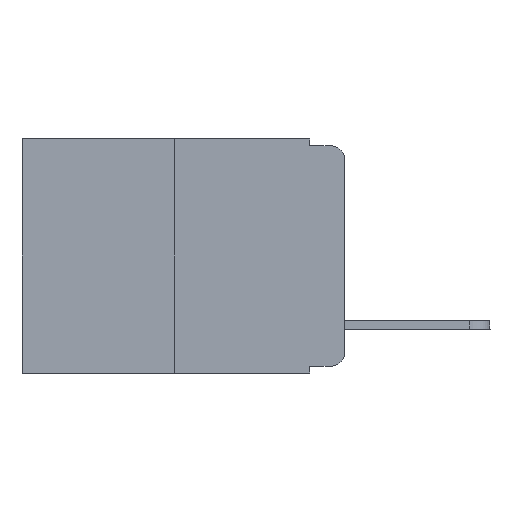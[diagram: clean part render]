
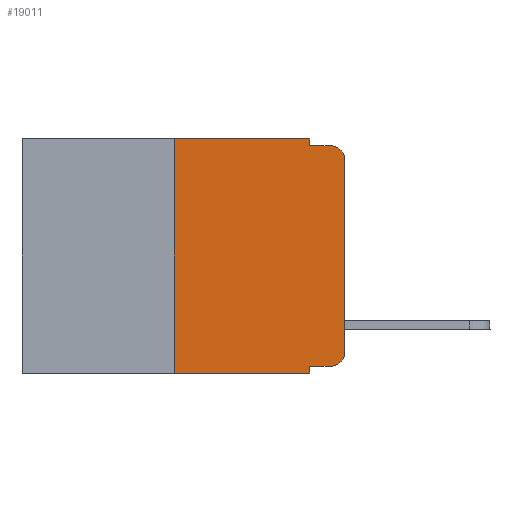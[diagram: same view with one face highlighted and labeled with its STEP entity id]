
A CAD part, left-side view. The second image highlights one B-rep face of the part: STEP entity #19011.
In plain terms, the highlighted planar face has unit normal (-1, 0, 0).
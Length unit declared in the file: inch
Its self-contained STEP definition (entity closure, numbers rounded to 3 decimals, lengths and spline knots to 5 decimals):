
#94 = VERTEX_POINT ( 'NONE', #7996 ) ;
#113 = EDGE_CURVE ( 'NONE', #15430, #3689, #9825, .T. ) ;
#119 = DIRECTION ( 'NONE',  ( -1., 0., 0. ) ) ;
#294 = DIRECTION ( 'NONE',  ( 0., 0., -1. ) ) ;
#566 = CARTESIAN_POINT ( 'NONE',  ( 0., 0.473, 0. ) ) ;
#1064 = ORIENTED_EDGE ( 'NONE', *, *, #1362, .F. ) ;
#1362 = EDGE_CURVE ( 'NONE', #15430, #94, #21019, .T. ) ;
#1914 = CIRCLE ( 'NONE', #5356, 0.02 ) ;
#1919 = CARTESIAN_POINT ( 'NONE',  ( 0., 0.051, 0. ) ) ;
#2071 = VECTOR ( 'NONE', #9882, 39.37008 ) ;
#2117 = VERTEX_POINT ( 'NONE', #2987 ) ;
#2472 = EDGE_CURVE ( 'NONE', #2117, #18087, #5117, .T. ) ;
#2649 = DIRECTION ( 'NONE',  ( 0., 0., 1. ) ) ;
#2950 = EDGE_CURVE ( 'NONE', #3612, #16257, #9960, .T. ) ;
#2987 = CARTESIAN_POINT ( 'NONE',  ( 0., 0.051, -0.01 ) ) ;
#3476 = DIRECTION ( 'NONE',  ( 0., 0., -1. ) ) ;
#3612 = VERTEX_POINT ( 'NONE', #15667 ) ;
#3689 = VERTEX_POINT ( 'NONE', #11002 ) ;
#3691 = VECTOR ( 'NONE', #4846, 39.37008 ) ;
#4055 = VECTOR ( 'NONE', #294, 39.37008 ) ;
#4326 = VECTOR ( 'NONE', #7541, 39.37008 ) ;
#4576 = CARTESIAN_POINT ( 'NONE',  ( 0., 0.473, 0. ) ) ;
#4703 = CARTESIAN_POINT ( 'NONE',  ( 0., 0.25, -0.343 ) ) ;
#4846 = DIRECTION ( 'NONE',  ( 0., -1., 0. ) ) ;
#5110 = EDGE_LOOP ( 'NONE', ( #17208, #15035, #13707, #11684, #19868, #1064, #16160, #17152, #14016, #7458 ) ) ;
#5117 = LINE ( 'NONE', #5328, #2071 ) ;
#5328 = CARTESIAN_POINT ( 'NONE',  ( 0., 0.051, -0.01 ) ) ;
#5356 = AXIS2_PLACEMENT_3D ( 'NONE', #14926, #119, #3476 ) ;
#6059 = CARTESIAN_POINT ( 'NONE',  ( 0., 0., -0.03 ) ) ;
#6173 = CARTESIAN_POINT ( 'NONE',  ( 0., 0.25, 0. ) ) ;
#6308 = EDGE_CURVE ( 'NONE', #16737, #3689, #9703, .T. ) ;
#6925 = LINE ( 'NONE', #566, #19804 ) ;
#7283 = VERTEX_POINT ( 'NONE', #10269 ) ;
#7458 = ORIENTED_EDGE ( 'NONE', *, *, #16545, .T. ) ;
#7541 = DIRECTION ( 'NONE',  ( 0., 0., -1. ) ) ;
#7996 = CARTESIAN_POINT ( 'NONE',  ( 0., 0.25, 0. ) ) ;
#9703 = LINE ( 'NONE', #1919, #4055 ) ;
#9825 = LINE ( 'NONE', #19689, #3691 ) ;
#9882 = DIRECTION ( 'NONE',  ( 0., -1., 0. ) ) ;
#9960 = LINE ( 'NONE', #10166, #10020 ) ;
#10020 = VECTOR ( 'NONE', #11370, 39.37008 ) ;
#10166 = CARTESIAN_POINT ( 'NONE',  ( 0., 0., 0. ) ) ;
#10269 = CARTESIAN_POINT ( 'NONE',  ( 0., 0.051, 0. ) ) ;
#10875 = EDGE_CURVE ( 'NONE', #7283, #2117, #17407, .T. ) ;
#11002 = CARTESIAN_POINT ( 'NONE',  ( 0., 0.051, -0.343 ) ) ;
#11277 = PLANE ( 'NONE',  #17519 ) ;
#11370 = DIRECTION ( 'NONE',  ( 0., 0., 1. ) ) ;
#11684 = ORIENTED_EDGE ( 'NONE', *, *, #10875, .F. ) ;
#11956 = VECTOR ( 'NONE', #13685, 39.37008 ) ;
#12162 = CARTESIAN_POINT ( 'NONE',  ( 0., 0.051, -0.333 ) ) ;
#12580 = DIRECTION ( 'NONE',  ( -1., 0., 0. ) ) ;
#13016 = EDGE_CURVE ( 'NONE', #16257, #18087, #15285, .T. ) ;
#13243 = EDGE_CURVE ( 'NONE', #94, #7283, #6925, .T. ) ;
#13685 = DIRECTION ( 'NONE',  ( 0., -1., 0. ) ) ;
#13707 = ORIENTED_EDGE ( 'NONE', *, *, #2472, .F. ) ;
#14016 = ORIENTED_EDGE ( 'NONE', *, *, #18840, .T. ) ;
#14196 = CARTESIAN_POINT ( 'NONE',  ( 0., 0.02, -0.03 ) ) ;
#14476 = CARTESIAN_POINT ( 'NONE',  ( 0., 0.02, -0.01 ) ) ;
#14798 = CARTESIAN_POINT ( 'NONE',  ( 0., 0.051, -0.333 ) ) ;
#14926 = CARTESIAN_POINT ( 'NONE',  ( 0., 0.02, -0.313 ) ) ;
#15035 = ORIENTED_EDGE ( 'NONE', *, *, #13016, .T. ) ;
#15285 = CIRCLE ( 'NONE', #16331, 0.02 ) ;
#15430 = VERTEX_POINT ( 'NONE', #4703 ) ;
#15667 = CARTESIAN_POINT ( 'NONE',  ( 0., 0., -0.313 ) ) ;
#16035 = DIRECTION ( 'NONE',  ( 0., 0., -1. ) ) ;
#16151 = DIRECTION ( 'NONE',  ( 1., 0., 0. ) ) ;
#16160 = ORIENTED_EDGE ( 'NONE', *, *, #113, .T. ) ;
#16257 = VERTEX_POINT ( 'NONE', #6059 ) ;
#16331 = AXIS2_PLACEMENT_3D ( 'NONE', #14196, #12580, #16035 ) ;
#16545 = EDGE_CURVE ( 'NONE', #19304, #3612, #1914, .T. ) ;
#16737 = VERTEX_POINT ( 'NONE', #14798 ) ;
#17152 = ORIENTED_EDGE ( 'NONE', *, *, #6308, .F. ) ;
#17208 = ORIENTED_EDGE ( 'NONE', *, *, #2950, .T. ) ;
#17369 = LINE ( 'NONE', #12162, #11956 ) ;
#17407 = LINE ( 'NONE', #19150, #4326 ) ;
#17519 = AXIS2_PLACEMENT_3D ( 'NONE', #4576, #16151, #17793 ) ;
#17548 = CARTESIAN_POINT ( 'NONE',  ( 0., 0.02, -0.333 ) ) ;
#17572 = FACE_OUTER_BOUND ( 'NONE', #5110, .T. ) ;
#17793 = DIRECTION ( 'NONE',  ( 0., 0., -1. ) ) ;
#18087 = VERTEX_POINT ( 'NONE', #14476 ) ;
#18706 = VECTOR ( 'NONE', #2649, 39.37008 ) ;
#18840 = EDGE_CURVE ( 'NONE', #16737, #19304, #17369, .T. ) ;
#19011 = ADVANCED_FACE ( 'NONE', ( #17572 ), #11277, .F. ) ;
#19150 = CARTESIAN_POINT ( 'NONE',  ( 0., 0.051, 0. ) ) ;
#19304 = VERTEX_POINT ( 'NONE', #17548 ) ;
#19689 = CARTESIAN_POINT ( 'NONE',  ( 0., 0.473, -0.343 ) ) ;
#19804 = VECTOR ( 'NONE', #20033, 39.37008 ) ;
#19868 = ORIENTED_EDGE ( 'NONE', *, *, #13243, .F. ) ;
#20033 = DIRECTION ( 'NONE',  ( 0., -1., 0. ) ) ;
#21019 = LINE ( 'NONE', #6173, #18706 ) ;
